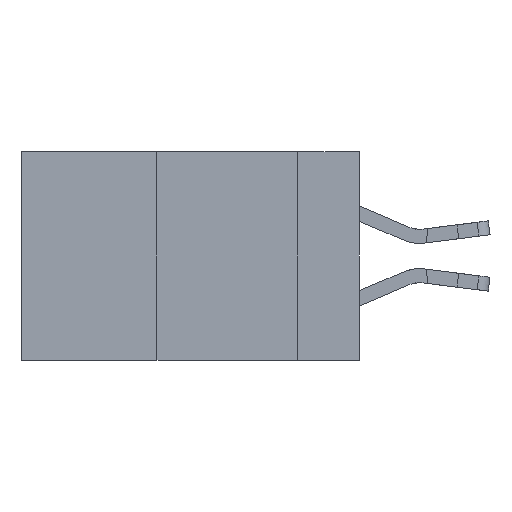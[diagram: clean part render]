
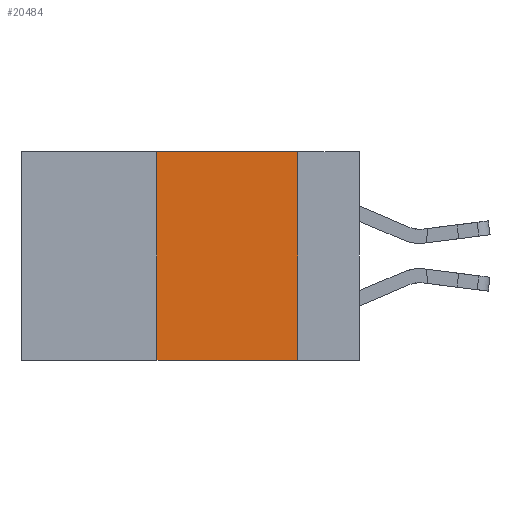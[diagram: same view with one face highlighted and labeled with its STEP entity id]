
A CAD part, left-side view. The second image highlights one B-rep face of the part: STEP entity #20484.
In plain terms, the highlighted planar face has unit normal (-1, 0, 0).
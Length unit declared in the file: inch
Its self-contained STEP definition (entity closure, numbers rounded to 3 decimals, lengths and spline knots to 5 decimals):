
#23 = VECTOR ( 'NONE', #22269, 39.37008 ) ;
#232 = CARTESIAN_POINT ( 'NONE',  ( 0., 0.11, 0. ) ) ;
#548 = VERTEX_POINT ( 'NONE', #1460 ) ;
#1460 = CARTESIAN_POINT ( 'NONE',  ( 0., 0.11, -0.37 ) ) ;
#1795 = ORIENTED_EDGE ( 'NONE', *, *, #19224, .F. ) ;
#1913 = DIRECTION ( 'NONE',  ( 0., 0., 1. ) ) ;
#2234 = VERTEX_POINT ( 'NONE', #232 ) ;
#2248 = DIRECTION ( 'NONE',  ( 0., -1., 0. ) ) ;
#2607 = CARTESIAN_POINT ( 'NONE',  ( 0., 0.36, 0. ) ) ;
#3776 = VECTOR ( 'NONE', #1913, 39.37008 ) ;
#5148 = CARTESIAN_POINT ( 'NONE',  ( 0., 0.36, -0.37 ) ) ;
#7700 = VECTOR ( 'NONE', #2248, 39.37008 ) ;
#7739 = AXIS2_PLACEMENT_3D ( 'NONE', #11602, #24175, #11333 ) ;
#7925 = EDGE_LOOP ( 'NONE', ( #9645, #1795, #10703, #10441 ) ) ;
#8019 = VERTEX_POINT ( 'NONE', #5148 ) ;
#8032 = DIRECTION ( 'NONE',  ( 0., -1., 0. ) ) ;
#9645 = ORIENTED_EDGE ( 'NONE', *, *, #23350, .F. ) ;
#10334 = CARTESIAN_POINT ( 'NONE',  ( 0., 0.6, -0.37 ) ) ;
#10441 = ORIENTED_EDGE ( 'NONE', *, *, #25316, .T. ) ;
#10703 = ORIENTED_EDGE ( 'NONE', *, *, #18863, .F. ) ;
#11309 = LINE ( 'NONE', #13601, #23 ) ;
#11333 = DIRECTION ( 'NONE',  ( 0., 0., -1. ) ) ;
#11602 = CARTESIAN_POINT ( 'NONE',  ( 0., 0.6, 0. ) ) ;
#13601 = CARTESIAN_POINT ( 'NONE',  ( 0., 0.11, 0. ) ) ;
#13815 = CARTESIAN_POINT ( 'NONE',  ( 0., 0.36, 0. ) ) ;
#15401 = VERTEX_POINT ( 'NONE', #2607 ) ;
#15909 = FACE_OUTER_BOUND ( 'NONE', #7925, .T. ) ;
#16437 = CARTESIAN_POINT ( 'NONE',  ( 0., 0.6, 0. ) ) ;
#18863 = EDGE_CURVE ( 'NONE', #8019, #15401, #22218, .T. ) ;
#19224 = EDGE_CURVE ( 'NONE', #15401, #2234, #20013, .T. ) ;
#19534 = VECTOR ( 'NONE', #8032, 39.37008 ) ;
#20013 = LINE ( 'NONE', #16437, #7700 ) ;
#20484 = ADVANCED_FACE ( 'NONE', ( #15909 ), #23909, .F. ) ;
#22218 = LINE ( 'NONE', #13815, #3776 ) ;
#22269 = DIRECTION ( 'NONE',  ( 0., 0., -1. ) ) ;
#22656 = LINE ( 'NONE', #10334, #19534 ) ;
#23350 = EDGE_CURVE ( 'NONE', #2234, #548, #11309, .T. ) ;
#23909 = PLANE ( 'NONE',  #7739 ) ;
#24175 = DIRECTION ( 'NONE',  ( 1., 0., 0. ) ) ;
#25316 = EDGE_CURVE ( 'NONE', #8019, #548, #22656, .T. ) ;
